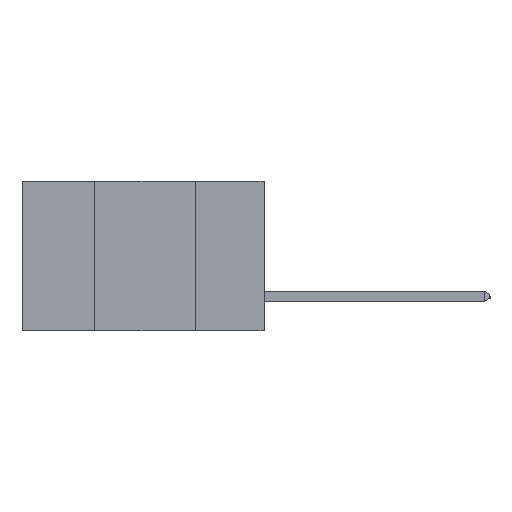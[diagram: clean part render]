
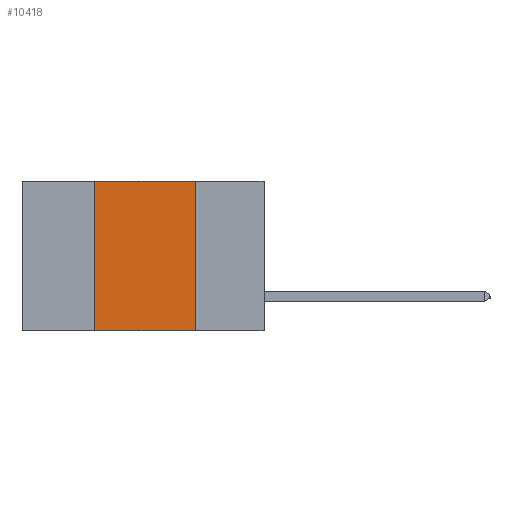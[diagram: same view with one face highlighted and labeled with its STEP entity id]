
A CAD part, left-side view. The second image highlights one B-rep face of the part: STEP entity #10418.
In plain terms, the highlighted planar face has unit normal (-1, 0, 0).
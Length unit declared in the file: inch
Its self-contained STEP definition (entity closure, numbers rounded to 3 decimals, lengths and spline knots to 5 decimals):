
#1238 = VECTOR ( 'NONE', #11573, 39.37008 ) ;
#2003 = VECTOR ( 'NONE', #17370, 39.37008 ) ;
#2650 = CARTESIAN_POINT ( 'NONE',  ( 0., 0.6, -0.37 ) ) ;
#2895 = DIRECTION ( 'NONE',  ( 0., 0., -1. ) ) ;
#3062 = DIRECTION ( 'NONE',  ( 0., 0., 1. ) ) ;
#4980 = VERTEX_POINT ( 'NONE', #15931 ) ;
#5018 = AXIS2_PLACEMENT_3D ( 'NONE', #20619, #8411, #25372 ) ;
#5057 = EDGE_CURVE ( 'NONE', #7256, #4980, #7714, .T. ) ;
#5490 = CARTESIAN_POINT ( 'NONE',  ( 0., 0.42, 0. ) ) ;
#5918 = PLANE ( 'NONE',  #5018 ) ;
#5919 = VERTEX_POINT ( 'NONE', #19395 ) ;
#6506 = ORIENTED_EDGE ( 'NONE', *, *, #30340, .F. ) ;
#7256 = VERTEX_POINT ( 'NONE', #28749 ) ;
#7714 = LINE ( 'NONE', #2650, #1238 ) ;
#8411 = DIRECTION ( 'NONE',  ( 1., 0., 0. ) ) ;
#10418 = ADVANCED_FACE ( 'NONE', ( #21609 ), #5918, .F. ) ;
#11573 = DIRECTION ( 'NONE',  ( 0., -1., 0. ) ) ;
#12964 = LINE ( 'NONE', #5490, #25036 ) ;
#15013 = LINE ( 'NONE', #29323, #2003 ) ;
#15339 = VECTOR ( 'NONE', #2895, 39.37008 ) ;
#15931 = CARTESIAN_POINT ( 'NONE',  ( 0., 0.17, -0.37 ) ) ;
#17370 = DIRECTION ( 'NONE',  ( 0., -1., 0. ) ) ;
#18060 = ORIENTED_EDGE ( 'NONE', *, *, #28027, .F. ) ;
#18165 = EDGE_CURVE ( 'NONE', #5919, #4980, #22551, .T. ) ;
#19269 = EDGE_LOOP ( 'NONE', ( #20686, #18060, #6506, #21070 ) ) ;
#19395 = CARTESIAN_POINT ( 'NONE',  ( 0., 0.17, 0. ) ) ;
#20029 = CARTESIAN_POINT ( 'NONE',  ( 0., 0.17, 0. ) ) ;
#20619 = CARTESIAN_POINT ( 'NONE',  ( 0., 0.6, 0. ) ) ;
#20686 = ORIENTED_EDGE ( 'NONE', *, *, #18165, .F. ) ;
#21070 = ORIENTED_EDGE ( 'NONE', *, *, #5057, .T. ) ;
#21609 = FACE_OUTER_BOUND ( 'NONE', #19269, .T. ) ;
#22551 = LINE ( 'NONE', #20029, #15339 ) ;
#23862 = CARTESIAN_POINT ( 'NONE',  ( 0., 0.42, 0. ) ) ;
#25036 = VECTOR ( 'NONE', #3062, 39.37008 ) ;
#25372 = DIRECTION ( 'NONE',  ( 0., 0., -1. ) ) ;
#28027 = EDGE_CURVE ( 'NONE', #31300, #5919, #15013, .T. ) ;
#28749 = CARTESIAN_POINT ( 'NONE',  ( 0., 0.42, -0.37 ) ) ;
#29323 = CARTESIAN_POINT ( 'NONE',  ( 0., 0.6, 0. ) ) ;
#30340 = EDGE_CURVE ( 'NONE', #7256, #31300, #12964, .T. ) ;
#31300 = VERTEX_POINT ( 'NONE', #23862 ) ;
